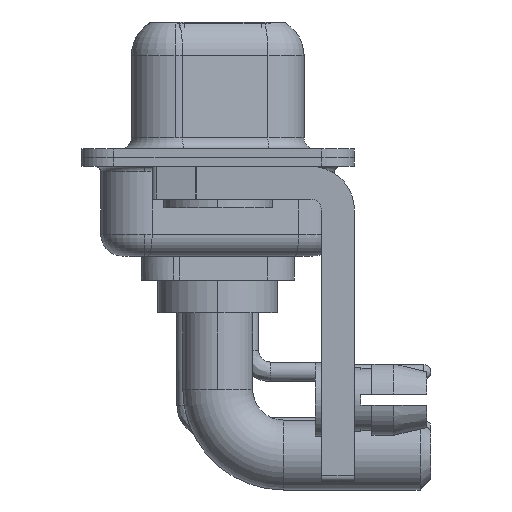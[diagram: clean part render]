
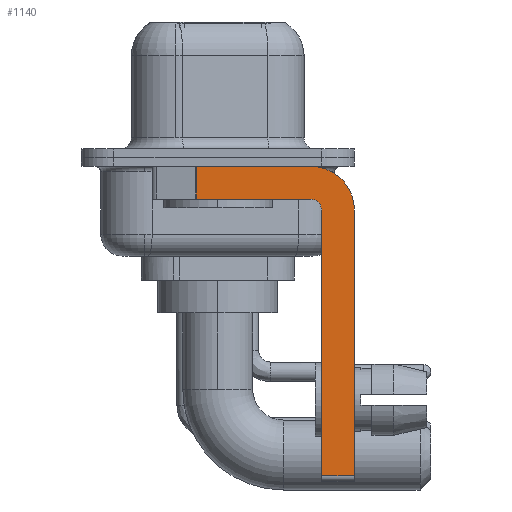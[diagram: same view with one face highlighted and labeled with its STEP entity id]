
A CAD part, left-side view. The second image highlights one B-rep face of the part: STEP entity #1140.
In plain terms, the highlighted planar face has unit normal (-1, 0, 0).
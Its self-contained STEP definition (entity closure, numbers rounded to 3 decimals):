
#99 = DIRECTION ( 'NONE',  ( 0., 0., -1. ) ) ;
#326 = VECTOR ( 'NONE', #21565, 1000. ) ;
#331 = CIRCLE ( 'NONE', #25745, 2. ) ;
#644 = DIRECTION ( 'NONE',  ( 1., 0., 0. ) ) ;
#938 = LINE ( 'NONE', #5416, #6424 ) ;
#939 = CARTESIAN_POINT ( 'NONE',  ( -2.9, -4.25, -0.4 ) ) ;
#1067 = DIRECTION ( 'NONE',  ( 0., -1., 0. ) ) ;
#1140 = ADVANCED_FACE ( 'NONE', ( #21183 ), #25019, .F. ) ;
#1224 = CARTESIAN_POINT ( 'NONE',  ( -2.9, -4.75, -14.8 ) ) ;
#1232 = ORIENTED_EDGE ( 'NONE', *, *, #17511, .F. ) ;
#1263 = CARTESIAN_POINT ( 'NONE',  ( -2.9, -4.25, -1.9 ) ) ;
#1553 = VERTEX_POINT ( 'NONE', #24854 ) ;
#1939 = CIRCLE ( 'NONE', #19311, 0.5 ) ;
#1957 = LINE ( 'NONE', #1224, #12535 ) ;
#2368 = VERTEX_POINT ( 'NONE', #17772 ) ;
#3340 = EDGE_CURVE ( 'NONE', #22119, #2368, #3885, .T. ) ;
#3356 = AXIS2_PLACEMENT_3D ( 'NONE', #20662, #644, #10949 ) ;
#3885 = LINE ( 'NONE', #20208, #17674 ) ;
#4025 = VERTEX_POINT ( 'NONE', #939 ) ;
#4766 = DIRECTION ( 'NONE',  ( 0., 0., 1. ) ) ;
#4798 = EDGE_CURVE ( 'NONE', #20323, #19834, #23670, .T. ) ;
#5416 = CARTESIAN_POINT ( 'NONE',  ( -2.9, 3., -0.4 ) ) ;
#6309 = ORIENTED_EDGE ( 'NONE', *, *, #24126, .F. ) ;
#6409 = ORIENTED_EDGE ( 'NONE', *, *, #3340, .T. ) ;
#6424 = VECTOR ( 'NONE', #1067, 1000. ) ;
#8608 = DIRECTION ( 'NONE',  ( 1., 0., 0. ) ) ;
#9197 = DIRECTION ( 'NONE',  ( 0., 1., 0. ) ) ;
#9657 = CARTESIAN_POINT ( 'NONE',  ( -2.9, -6.25, -2.4 ) ) ;
#10160 = LINE ( 'NONE', #18235, #11619 ) ;
#10343 = EDGE_CURVE ( 'NONE', #14729, #19834, #10160, .T. ) ;
#10949 = DIRECTION ( 'NONE',  ( 0., 0., -1. ) ) ;
#11379 = CARTESIAN_POINT ( 'NONE',  ( -2.9, -4.25, -1.9 ) ) ;
#11619 = VECTOR ( 'NONE', #99, 1000. ) ;
#11656 = VERTEX_POINT ( 'NONE', #9657 ) ;
#12535 = VECTOR ( 'NONE', #18120, 1000. ) ;
#13857 = EDGE_CURVE ( 'NONE', #4025, #11656, #331, .T. ) ;
#14219 = ORIENTED_EDGE ( 'NONE', *, *, #24963, .F. ) ;
#14729 = VERTEX_POINT ( 'NONE', #15363 ) ;
#14825 = CARTESIAN_POINT ( 'NONE',  ( -2.9, -4.25, -2.4 ) ) ;
#15363 = CARTESIAN_POINT ( 'NONE',  ( -2.9, 0.978, -0.4 ) ) ;
#17511 = EDGE_CURVE ( 'NONE', #14729, #4025, #938, .T. ) ;
#17554 = CARTESIAN_POINT ( 'NONE',  ( -2.9, -6.25, -2.4 ) ) ;
#17674 = VECTOR ( 'NONE', #22324, 1000. ) ;
#17772 = CARTESIAN_POINT ( 'NONE',  ( -2.9, -6.25, -14.55 ) ) ;
#18120 = DIRECTION ( 'NONE',  ( 0., 0., 1. ) ) ;
#18235 = CARTESIAN_POINT ( 'NONE',  ( -2.9, 0.978, -1.9 ) ) ;
#18596 = CARTESIAN_POINT ( 'NONE',  ( -2.9, 0.978, -1.9 ) ) ;
#18817 = CARTESIAN_POINT ( 'NONE',  ( -2.9, -4.75, -14.55 ) ) ;
#19070 = DIRECTION ( 'NONE',  ( 0., 0., -1. ) ) ;
#19311 = AXIS2_PLACEMENT_3D ( 'NONE', #14825, #22949, #4766 ) ;
#19834 = VERTEX_POINT ( 'NONE', #18596 ) ;
#20208 = CARTESIAN_POINT ( 'NONE',  ( -2.9, -4.25, -14.55 ) ) ;
#20323 = VERTEX_POINT ( 'NONE', #11379 ) ;
#20553 = CARTESIAN_POINT ( 'NONE',  ( -2.9, -4.25, -2.4 ) ) ;
#20662 = CARTESIAN_POINT ( 'NONE',  ( -2.9, -4.25, -2.4 ) ) ;
#21183 = FACE_OUTER_BOUND ( 'NONE', #25675, .T. ) ;
#21565 = DIRECTION ( 'NONE',  ( 0., 0., -1. ) ) ;
#21570 = ORIENTED_EDGE ( 'NONE', *, *, #4798, .F. ) ;
#22119 = VERTEX_POINT ( 'NONE', #18817 ) ;
#22324 = DIRECTION ( 'NONE',  ( 0., -1., 0. ) ) ;
#22475 = VECTOR ( 'NONE', #9197, 1000. ) ;
#22696 = EDGE_CURVE ( 'NONE', #1553, #20323, #1939, .T. ) ;
#22949 = DIRECTION ( 'NONE',  ( -1., 0., 0. ) ) ;
#23670 = LINE ( 'NONE', #1263, #22475 ) ;
#24126 = EDGE_CURVE ( 'NONE', #11656, #2368, #26053, .T. ) ;
#24278 = ORIENTED_EDGE ( 'NONE', *, *, #13857, .F. ) ;
#24854 = CARTESIAN_POINT ( 'NONE',  ( -2.9, -4.75, -2.4 ) ) ;
#24963 = EDGE_CURVE ( 'NONE', #22119, #1553, #1957, .T. ) ;
#25019 = PLANE ( 'NONE',  #3356 ) ;
#25147 = ORIENTED_EDGE ( 'NONE', *, *, #10343, .T. ) ;
#25297 = ORIENTED_EDGE ( 'NONE', *, *, #22696, .F. ) ;
#25675 = EDGE_LOOP ( 'NONE', ( #1232, #25147, #21570, #25297, #14219, #6409, #6309, #24278 ) ) ;
#25745 = AXIS2_PLACEMENT_3D ( 'NONE', #20553, #8608, #19070 ) ;
#26053 = LINE ( 'NONE', #17554, #326 ) ;
